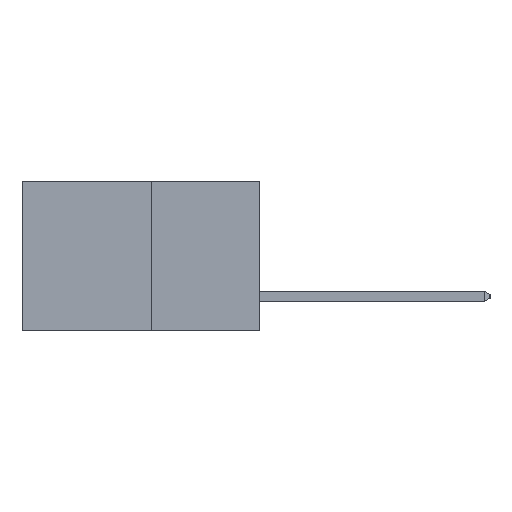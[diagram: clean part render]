
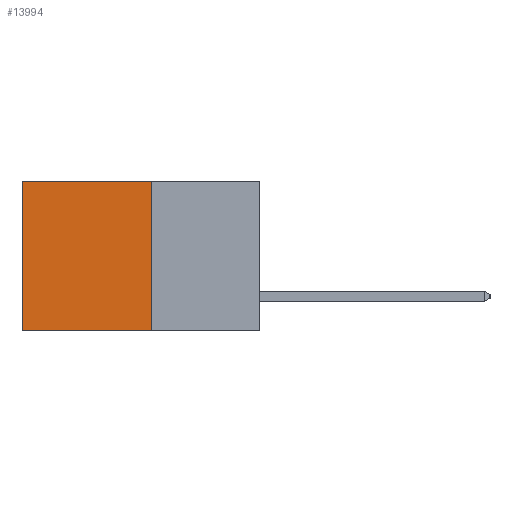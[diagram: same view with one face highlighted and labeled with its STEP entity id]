
A CAD part, left-side view. The second image highlights one B-rep face of the part: STEP entity #13994.
In plain terms, the highlighted planar face has unit normal (-1, 0, 0).
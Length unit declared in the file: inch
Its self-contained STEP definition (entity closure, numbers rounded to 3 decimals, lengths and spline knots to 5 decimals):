
#228 = CARTESIAN_POINT ( 'NONE',  ( 0.277, 0.27, -0.37 ) ) ;
#383 = EDGE_LOOP ( 'NONE', ( #18251, #10160, #10661, #4509 ) ) ;
#1856 = PLANE ( 'NONE',  #13423 ) ;
#2176 = CARTESIAN_POINT ( 'NONE',  ( 0.277, 0.27, -0.37 ) ) ;
#3481 = DIRECTION ( 'NONE',  ( 1., 0., 0. ) ) ;
#3974 = LINE ( 'NONE', #4508, #16074 ) ;
#4508 = CARTESIAN_POINT ( 'NONE',  ( 0.277, 0.27, 0. ) ) ;
#4509 = ORIENTED_EDGE ( 'NONE', *, *, #13094, .T. ) ;
#4802 = CARTESIAN_POINT ( 'NONE',  ( 0.277, 0.27, 0. ) ) ;
#6336 = EDGE_CURVE ( 'NONE', #19562, #15219, #9951, .T. ) ;
#6341 = DIRECTION ( 'NONE',  ( 0., 0., -1. ) ) ;
#9575 = CARTESIAN_POINT ( 'NONE',  ( 0.277, 0.27, -0.37 ) ) ;
#9951 = LINE ( 'NONE', #19165, #17795 ) ;
#10160 = ORIENTED_EDGE ( 'NONE', *, *, #6336, .F. ) ;
#10488 = VECTOR ( 'NONE', #6341, 39.37008 ) ;
#10661 = ORIENTED_EDGE ( 'NONE', *, *, #17517, .F. ) ;
#10677 = CARTESIAN_POINT ( 'NONE',  ( 0.277, 0.59, -0.37 ) ) ;
#11426 = DIRECTION ( 'NONE',  ( 0., 1., 0. ) ) ;
#11472 = LINE ( 'NONE', #9575, #10488 ) ;
#12257 = LINE ( 'NONE', #10677, #20068 ) ;
#13094 = EDGE_CURVE ( 'NONE', #17520, #19791, #3974, .T. ) ;
#13423 = AXIS2_PLACEMENT_3D ( 'NONE', #228, #3481, #14575 ) ;
#13994 = ADVANCED_FACE ( 'NONE', ( #19196 ), #1856, .F. ) ;
#14575 = DIRECTION ( 'NONE',  ( 0., 0., -1. ) ) ;
#15219 = VERTEX_POINT ( 'NONE', #17856 ) ;
#15556 = DIRECTION ( 'NONE',  ( 0., 1., 0. ) ) ;
#16074 = VECTOR ( 'NONE', #15556, 39.37008 ) ;
#16765 = EDGE_CURVE ( 'NONE', #19791, #15219, #12257, .T. ) ;
#16819 = CARTESIAN_POINT ( 'NONE',  ( 0.277, 0.59, 0. ) ) ;
#17517 = EDGE_CURVE ( 'NONE', #17520, #19562, #11472, .T. ) ;
#17520 = VERTEX_POINT ( 'NONE', #4802 ) ;
#17795 = VECTOR ( 'NONE', #11426, 39.37008 ) ;
#17856 = CARTESIAN_POINT ( 'NONE',  ( 0.277, 0.59, -0.37 ) ) ;
#18251 = ORIENTED_EDGE ( 'NONE', *, *, #16765, .T. ) ;
#19165 = CARTESIAN_POINT ( 'NONE',  ( 0.277, 0.27, -0.37 ) ) ;
#19196 = FACE_OUTER_BOUND ( 'NONE', #383, .T. ) ;
#19562 = VERTEX_POINT ( 'NONE', #2176 ) ;
#19791 = VERTEX_POINT ( 'NONE', #16819 ) ;
#20047 = DIRECTION ( 'NONE',  ( 0., 0., -1. ) ) ;
#20068 = VECTOR ( 'NONE', #20047, 39.37008 ) ;
